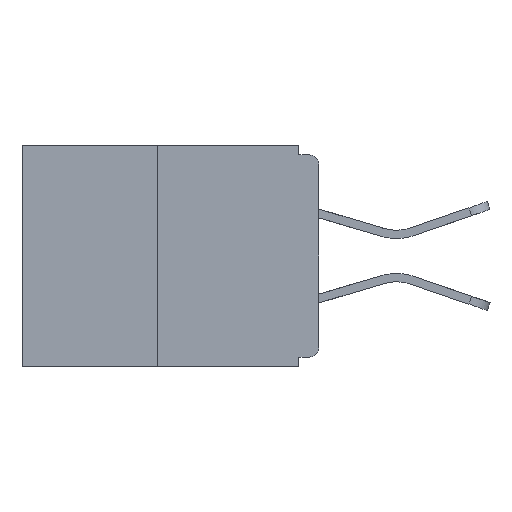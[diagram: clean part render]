
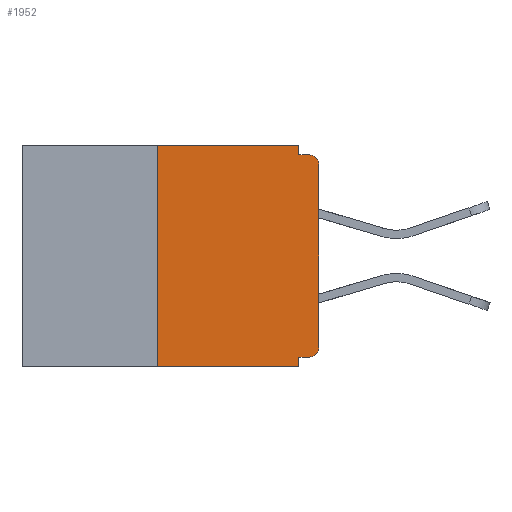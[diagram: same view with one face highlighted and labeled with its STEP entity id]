
A CAD part, left-side view. The second image highlights one B-rep face of the part: STEP entity #1952.
In plain terms, the highlighted planar face has unit normal (-1, 0, 0).
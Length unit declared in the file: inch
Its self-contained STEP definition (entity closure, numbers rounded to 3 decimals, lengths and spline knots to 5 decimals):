
#30 = VECTOR ( 'NONE', #13053, 39.37008 ) ;
#266 = VERTEX_POINT ( 'NONE', #6878 ) ;
#281 = ORIENTED_EDGE ( 'NONE', *, *, #13738, .F. ) ;
#527 = EDGE_CURVE ( 'NONE', #266, #3989, #7795, .T. ) ;
#901 = VECTOR ( 'NONE', #911, 39.37008 ) ;
#911 = DIRECTION ( 'NONE',  ( 0., 0., -1. ) ) ;
#1119 = LINE ( 'NONE', #10377, #901 ) ;
#1121 = LINE ( 'NONE', #14258, #3855 ) ;
#1450 = EDGE_CURVE ( 'NONE', #13347, #2103, #20283, .T. ) ;
#1501 = DIRECTION ( 'NONE',  ( -1., 0., 0. ) ) ;
#1673 = DIRECTION ( 'NONE',  ( 0., -1., 0. ) ) ;
#1789 = CIRCLE ( 'NONE', #19873, 0.015 ) ;
#1900 = VERTEX_POINT ( 'NONE', #6633 ) ;
#1952 = ADVANCED_FACE ( 'NONE', ( #6014 ), #16599, .F. ) ;
#2103 = VERTEX_POINT ( 'NONE', #12800 ) ;
#2250 = VECTOR ( 'NONE', #3936, 39.37008 ) ;
#2417 = DIRECTION ( 'NONE',  ( 0., 0., -1. ) ) ;
#2578 = VERTEX_POINT ( 'NONE', #2845 ) ;
#2597 = EDGE_CURVE ( 'NONE', #17733, #7919, #1789, .T. ) ;
#2739 = EDGE_CURVE ( 'NONE', #7296, #3989, #4243, .T. ) ;
#2845 = CARTESIAN_POINT ( 'NONE',  ( 0., 0.031, 0. ) ) ;
#2889 = ORIENTED_EDGE ( 'NONE', *, *, #18534, .F. ) ;
#3802 = AXIS2_PLACEMENT_3D ( 'NONE', #18294, #15082, #2417 ) ;
#3855 = VECTOR ( 'NONE', #11157, 39.37008 ) ;
#3869 = CARTESIAN_POINT ( 'NONE',  ( 0., 0.25, 0. ) ) ;
#3936 = DIRECTION ( 'NONE',  ( 0., 0., 1. ) ) ;
#3989 = VERTEX_POINT ( 'NONE', #11521 ) ;
#4241 = VECTOR ( 'NONE', #11881, 39.37008 ) ;
#4243 = LINE ( 'NONE', #17436, #30 ) ;
#4715 = DIRECTION ( 'NONE',  ( -1., 0., 0. ) ) ;
#4828 = ORIENTED_EDGE ( 'NONE', *, *, #12772, .F. ) ;
#4889 = ORIENTED_EDGE ( 'NONE', *, *, #14226, .T. ) ;
#5324 = CARTESIAN_POINT ( 'NONE',  ( 0., 0.46, 0. ) ) ;
#5538 = CARTESIAN_POINT ( 'NONE',  ( 0., 0., 0. ) ) ;
#5735 = LINE ( 'NONE', #5538, #4241 ) ;
#6014 = FACE_OUTER_BOUND ( 'NONE', #16423, .T. ) ;
#6212 = EDGE_CURVE ( 'NONE', #17733, #7296, #1121, .T. ) ;
#6371 = DIRECTION ( 'NONE',  ( 0., 0., -1. ) ) ;
#6633 = CARTESIAN_POINT ( 'NONE',  ( 0., 0.25, 0. ) ) ;
#6689 = CARTESIAN_POINT ( 'NONE',  ( 0., 0.031, -0.328 ) ) ;
#6766 = DIRECTION ( 'NONE',  ( 0., -1., 0. ) ) ;
#6878 = CARTESIAN_POINT ( 'NONE',  ( 0., 0.25, -0.343 ) ) ;
#7296 = VERTEX_POINT ( 'NONE', #6689 ) ;
#7743 = DIRECTION ( 'NONE',  ( 0., -1., 0. ) ) ;
#7795 = LINE ( 'NONE', #20165, #12005 ) ;
#7919 = VERTEX_POINT ( 'NONE', #13419 ) ;
#9239 = VECTOR ( 'NONE', #6766, 39.37008 ) ;
#9617 = CARTESIAN_POINT ( 'NONE',  ( 0., 0., -0.015 ) ) ;
#10341 = AXIS2_PLACEMENT_3D ( 'NONE', #18568, #1501, #12521 ) ;
#10377 = CARTESIAN_POINT ( 'NONE',  ( 0., 0.031, 0. ) ) ;
#11157 = DIRECTION ( 'NONE',  ( 0., 1., 0. ) ) ;
#11376 = CARTESIAN_POINT ( 'NONE',  ( 0., 0.031, -0.015 ) ) ;
#11521 = CARTESIAN_POINT ( 'NONE',  ( 0., 0.031, -0.343 ) ) ;
#11881 = DIRECTION ( 'NONE',  ( 0., 0., 1. ) ) ;
#11885 = ORIENTED_EDGE ( 'NONE', *, *, #2739, .F. ) ;
#12005 = VECTOR ( 'NONE', #7743, 39.37008 ) ;
#12430 = VECTOR ( 'NONE', #1673, 39.37008 ) ;
#12521 = DIRECTION ( 'NONE',  ( 0., 0., -1. ) ) ;
#12767 = CARTESIAN_POINT ( 'NONE',  ( 0., 0., -0.03 ) ) ;
#12772 = EDGE_CURVE ( 'NONE', #266, #1900, #15308, .T. ) ;
#12800 = CARTESIAN_POINT ( 'NONE',  ( 0., 0.015, -0.015 ) ) ;
#13053 = DIRECTION ( 'NONE',  ( 0., 0., -1. ) ) ;
#13347 = VERTEX_POINT ( 'NONE', #11376 ) ;
#13419 = CARTESIAN_POINT ( 'NONE',  ( 0., 0., -0.313 ) ) ;
#13738 = EDGE_CURVE ( 'NONE', #1900, #2578, #14647, .T. ) ;
#13829 = ORIENTED_EDGE ( 'NONE', *, *, #6212, .F. ) ;
#14068 = ORIENTED_EDGE ( 'NONE', *, *, #15376, .T. ) ;
#14167 = CARTESIAN_POINT ( 'NONE',  ( 0., 0.015, -0.313 ) ) ;
#14226 = EDGE_CURVE ( 'NONE', #15683, #2103, #14388, .T. ) ;
#14258 = CARTESIAN_POINT ( 'NONE',  ( 0., 0., -0.328 ) ) ;
#14360 = CARTESIAN_POINT ( 'NONE',  ( 0., 0.015, -0.328 ) ) ;
#14388 = CIRCLE ( 'NONE', #10341, 0.015 ) ;
#14647 = LINE ( 'NONE', #5324, #9239 ) ;
#15082 = DIRECTION ( 'NONE',  ( 1., 0., 0. ) ) ;
#15308 = LINE ( 'NONE', #3869, #2250 ) ;
#15376 = EDGE_CURVE ( 'NONE', #7919, #15683, #5735, .T. ) ;
#15683 = VERTEX_POINT ( 'NONE', #12767 ) ;
#16423 = EDGE_LOOP ( 'NONE', ( #281, #4828, #17042, #11885, #13829, #18926, #14068, #4889, #18564, #2889 ) ) ;
#16599 = PLANE ( 'NONE',  #3802 ) ;
#17042 = ORIENTED_EDGE ( 'NONE', *, *, #527, .T. ) ;
#17436 = CARTESIAN_POINT ( 'NONE',  ( 0., 0.031, -0.343 ) ) ;
#17733 = VERTEX_POINT ( 'NONE', #14360 ) ;
#18294 = CARTESIAN_POINT ( 'NONE',  ( 0., 0.46, 0. ) ) ;
#18534 = EDGE_CURVE ( 'NONE', #2578, #13347, #1119, .T. ) ;
#18564 = ORIENTED_EDGE ( 'NONE', *, *, #1450, .F. ) ;
#18568 = CARTESIAN_POINT ( 'NONE',  ( 0., 0.015, -0.03 ) ) ;
#18926 = ORIENTED_EDGE ( 'NONE', *, *, #2597, .T. ) ;
#19873 = AXIS2_PLACEMENT_3D ( 'NONE', #14167, #4715, #6371 ) ;
#20165 = CARTESIAN_POINT ( 'NONE',  ( 0., 0.46, -0.343 ) ) ;
#20283 = LINE ( 'NONE', #9617, #12430 ) ;
